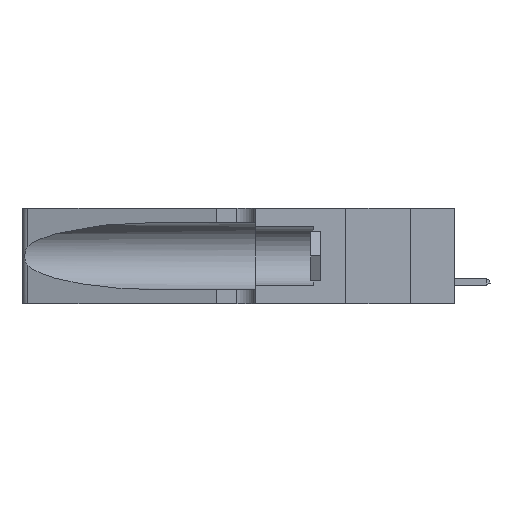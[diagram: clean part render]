
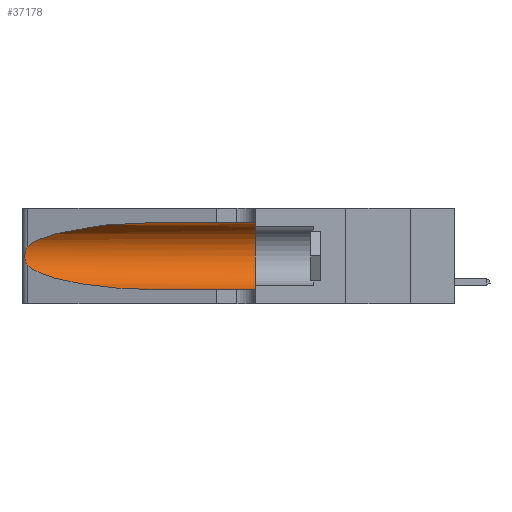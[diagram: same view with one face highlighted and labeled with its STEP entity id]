
A CAD part, left-side view. The second image highlights one B-rep face of the part: STEP entity #37178.
In plain terms, the highlighted cylindrical face has radius 3.308 mm (diameter 6.617 mm), a partial arc.
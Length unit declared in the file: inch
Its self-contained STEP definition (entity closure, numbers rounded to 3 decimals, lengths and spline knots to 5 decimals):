
#515 = ORIENTED_EDGE ( 'NONE', *, *, #27955, .T. ) ;
#732 = EDGE_LOOP ( 'NONE', ( #18443, #515, #17901, #33440, #30525, #42673 ) ) ;
#1031 = VERTEX_POINT ( 'NONE', #24178 ) ;
#1550 = CARTESIAN_POINT ( 'NONE',  ( 0.1305, 0.72297, 0.31525 ) ) ;
#1826 = VERTEX_POINT ( 'NONE', #32237 ) ;
#1849 = VECTOR ( 'NONE', #45210, 39.37008 ) ;
#2737 = DIRECTION ( 'NONE',  ( 0., -1., 0. ) ) ;
#3013 = CARTESIAN_POINT ( 'NONE',  ( 0.1305, 0.72297, 0.31525 ) ) ;
#3238 = EDGE_CURVE ( 'NONE', #36636, #47917, #8671, .T. ) ;
#3253 = CARTESIAN_POINT ( 'NONE',  ( 0.25487, 1.22718, 0.22369 ) ) ;
#6306 = VERTEX_POINT ( 'NONE', #6409 ) ;
#6409 = CARTESIAN_POINT ( 'NONE',  ( 0.1305, 0.35, 0.31525 ) ) ;
#6497 = CARTESIAN_POINT ( 'NONE',  ( 0.25639, 1.23184, 0.21858 ) ) ;
#8076 = EDGE_CURVE ( 'NONE', #36636, #6306, #33130, .T. ) ;
#8480 = AXIS2_PLACEMENT_3D ( 'NONE', #24648, #2737, #18157 ) ;
#8671 =( BOUNDED_CURVE ( )  B_SPLINE_CURVE ( 3, ( #3013, #25753, #32754, #40552 ),
 .UNSPECIFIED., .F., .F. ) 
 B_SPLINE_CURVE_WITH_KNOTS ( ( 4, 4 ),
 ( 1.5708, 2.84003 ),
 .UNSPECIFIED. ) 
 CURVE ( )  GEOMETRIC_REPRESENTATION_ITEM ( )  RATIONAL_B_SPLINE_CURVE ( ( 1., 0.87, 0.87, 1. ) ) 
 REPRESENTATION_ITEM ( '' )  );
#10087 = CARTESIAN_POINT ( 'NONE',  ( 0.18966, 0.96281, 0.05475 ) ) ;
#10140 = CARTESIAN_POINT ( 'NONE',  ( 0.25487, 1.22718, 0.14631 ) ) ;
#13663 = CARTESIAN_POINT ( 'NONE',  ( 0.25555, 1.22994, 0.2215 ) ) ;
#13977 = CARTESIAN_POINT ( 'NONE',  ( 0.25854, 1.2359, 0.20912 ) ) ;
#17371 = CARTESIAN_POINT ( 'NONE',  ( 0.25856, 1.23593, 0.16098 ) ) ;
#17901 = ORIENTED_EDGE ( 'NONE', *, *, #19587, .T. ) ;
#18157 = DIRECTION ( 'NONE',  ( 0., 0., -1. ) ) ;
#18385 = AXIS2_PLACEMENT_3D ( 'NONE', #22842, #30293, #30457 ) ;
#18443 = ORIENTED_EDGE ( 'NONE', *, *, #3238, .T. ) ;
#18644 = CARTESIAN_POINT ( 'NONE',  ( 0.25555, 1.22993, 0.14849 ) ) ;
#19587 = EDGE_CURVE ( 'NONE', #20672, #1031, #41137, .T. ) ;
#20265 = DIRECTION ( 'NONE',  ( 0., -1., 0. ) ) ;
#20672 = VERTEX_POINT ( 'NONE', #10140 ) ;
#21153 = EDGE_CURVE ( 'NONE', #1031, #1826, #26231, .T. ) ;
#21448 = CARTESIAN_POINT ( 'NONE',  ( 0.26018, 1.23835, 0.19895 ) ) ;
#21874 = EDGE_CURVE ( 'NONE', #6306, #1826, #34682, .T. ) ;
#22393 = B_SPLINE_CURVE_WITH_KNOTS ( 'NONE', 3,
 ( #3253, #13663, #6497, #39805, #13977, #21448, #47389, #35941, #25163, #17371, #25328, #47070, #18644, #37061 ),
 .UNSPECIFIED., .F., .F.,
 ( 4, 2, 2, 2, 2, 2, 4 ),
 ( 0., 0.00027, 0.00053, 0.00107, 0.0016, 0.00187, 0.00214 ),
 .UNSPECIFIED. ) ;
#22842 = CARTESIAN_POINT ( 'NONE',  ( 0.1305, 0.35, 0.185 ) ) ;
#22847 = CARTESIAN_POINT ( 'NONE',  ( 0.1305, 1.61858, 0.05475 ) ) ;
#23019 = CYLINDRICAL_SURFACE ( 'NONE', #8480, 0.13025 ) ;
#24178 = CARTESIAN_POINT ( 'NONE',  ( 0.1305, 0.72297, 0.05475 ) ) ;
#24648 = CARTESIAN_POINT ( 'NONE',  ( 0.1305, 1.61858, 0.185 ) ) ;
#25163 = CARTESIAN_POINT ( 'NONE',  ( 0.26017, 1.23833, 0.17102 ) ) ;
#25328 = CARTESIAN_POINT ( 'NONE',  ( 0.25789, 1.23486, 0.15765 ) ) ;
#25753 = CARTESIAN_POINT ( 'NONE',  ( 0.18966, 0.96281, 0.31525 ) ) ;
#25822 = CARTESIAN_POINT ( 'NONE',  ( 0.1305, 0.72297, 0.05475 ) ) ;
#26231 = LINE ( 'NONE', #22847, #1849 ) ;
#27093 = CARTESIAN_POINT ( 'NONE',  ( 0.1305, 1.61858, 0.31525 ) ) ;
#27955 = EDGE_CURVE ( 'NONE', #47917, #20672, #22393, .T. ) ;
#30293 = DIRECTION ( 'NONE',  ( 0., 1., 0. ) ) ;
#30457 = DIRECTION ( 'NONE',  ( 0., 0., 1. ) ) ;
#30525 = ORIENTED_EDGE ( 'NONE', *, *, #21874, .F. ) ;
#32237 = CARTESIAN_POINT ( 'NONE',  ( 0.1305, 0.35, 0.05475 ) ) ;
#32754 = CARTESIAN_POINT ( 'NONE',  ( 0.2373, 1.15595, 0.28018 ) ) ;
#33130 = LINE ( 'NONE', #27093, #40695 ) ;
#33440 = ORIENTED_EDGE ( 'NONE', *, *, #21153, .T. ) ;
#34682 = CIRCLE ( 'NONE', #18385, 0.13025 ) ;
#35260 = FACE_OUTER_BOUND ( 'NONE', #732, .T. ) ;
#35941 = CARTESIAN_POINT ( 'NONE',  ( 0.26075, 1.23896, 0.178 ) ) ;
#36636 = VERTEX_POINT ( 'NONE', #1550 ) ;
#37061 = CARTESIAN_POINT ( 'NONE',  ( 0.25487, 1.22718, 0.14631 ) ) ;
#37178 = ADVANCED_FACE ( 'NONE', ( #35260 ), #23019, .F. ) ;
#39805 = CARTESIAN_POINT ( 'NONE',  ( 0.25787, 1.23484, 0.2124 ) ) ;
#40552 = CARTESIAN_POINT ( 'NONE',  ( 0.25487, 1.22718, 0.22369 ) ) ;
#40695 = VECTOR ( 'NONE', #20265, 39.37008 ) ;
#41135 = CARTESIAN_POINT ( 'NONE',  ( 0.25487, 1.22718, 0.14631 ) ) ;
#41137 =( BOUNDED_CURVE ( )  B_SPLINE_CURVE ( 3, ( #41135, #42615, #10087, #25822 ),
 .UNSPECIFIED., .F., .F. ) 
 B_SPLINE_CURVE_WITH_KNOTS ( ( 4, 4 ),
 ( 3.44316, 4.71239 ),
 .UNSPECIFIED. ) 
 CURVE ( )  GEOMETRIC_REPRESENTATION_ITEM ( )  RATIONAL_B_SPLINE_CURVE ( ( 1., 0.87, 0.87, 1. ) ) 
 REPRESENTATION_ITEM ( '' )  );
#42615 = CARTESIAN_POINT ( 'NONE',  ( 0.2373, 1.15595, 0.08982 ) ) ;
#42673 = ORIENTED_EDGE ( 'NONE', *, *, #8076, .F. ) ;
#45210 = DIRECTION ( 'NONE',  ( 0., -1., 0. ) ) ;
#47070 = CARTESIAN_POINT ( 'NONE',  ( 0.25639, 1.23186, 0.15144 ) ) ;
#47259 = CARTESIAN_POINT ( 'NONE',  ( 0.25487, 1.22718, 0.22369 ) ) ;
#47389 = CARTESIAN_POINT ( 'NONE',  ( 0.26075, 1.23896, 0.19203 ) ) ;
#47917 = VERTEX_POINT ( 'NONE', #47259 ) ;
